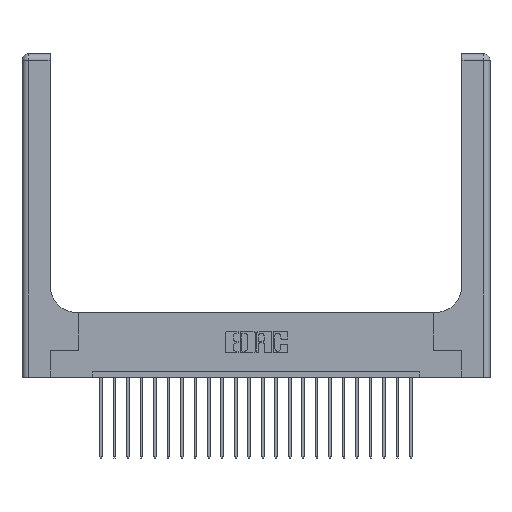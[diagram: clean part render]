
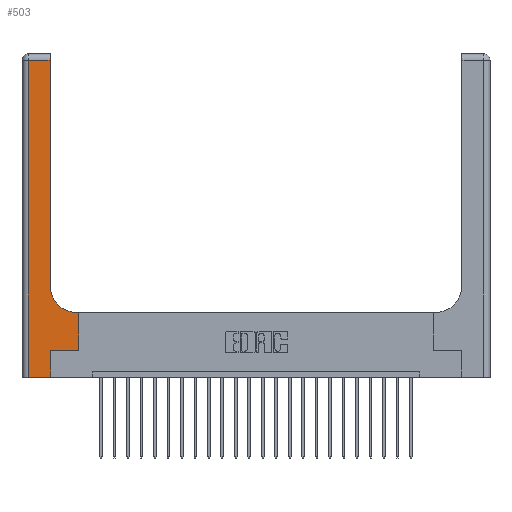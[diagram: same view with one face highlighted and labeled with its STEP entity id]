
A CAD part, top view. The second image highlights one B-rep face of the part: STEP entity #503.
In plain terms, the highlighted planar face has unit normal (0, 0, 1).
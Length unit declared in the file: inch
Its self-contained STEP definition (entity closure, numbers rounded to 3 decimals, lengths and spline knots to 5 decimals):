
#93 = LINE ( 'NONE', #9134, #2619 ) ;
#501 = FACE_OUTER_BOUND ( 'NONE', #10092, .T. ) ;
#503 = ADVANCED_FACE ( 'NONE', ( #501 ), #2582, .F. ) ;
#717 = VERTEX_POINT ( 'NONE', #13476 ) ;
#799 = ORIENTED_EDGE ( 'NONE', *, *, #3414, .T. ) ;
#1253 = CARTESIAN_POINT ( 'NONE',  ( 0.26, 2.94, 0.37 ) ) ;
#1261 = DIRECTION ( 'NONE',  ( 0., 1., 0. ) ) ;
#1490 = LINE ( 'NONE', #8557, #13143 ) ;
#2034 = VERTEX_POINT ( 'NONE', #3528 ) ;
#2071 = ORIENTED_EDGE ( 'NONE', *, *, #3049, .T. ) ;
#2171 = VECTOR ( 'NONE', #18870, 39.37008 ) ;
#2581 = VECTOR ( 'NONE', #14465, 39.37008 ) ;
#2582 = PLANE ( 'NONE',  #10431 ) ;
#2619 = VECTOR ( 'NONE', #10775, 39.37008 ) ;
#2918 = AXIS2_PLACEMENT_3D ( 'NONE', #22586, #13736, #18854 ) ;
#3049 = EDGE_CURVE ( 'NONE', #10993, #2034, #16896, .T. ) ;
#3401 = ORIENTED_EDGE ( 'NONE', *, *, #21704, .T. ) ;
#3414 = EDGE_CURVE ( 'NONE', #13813, #12497, #21888, .T. ) ;
#3528 = CARTESIAN_POINT ( 'NONE',  ( 0.06, 2.94, 0.37 ) ) ;
#3960 = EDGE_CURVE ( 'NONE', #717, #10993, #1490, .T. ) ;
#4150 = DIRECTION ( 'NONE',  ( 0., 1., 0. ) ) ;
#4334 = EDGE_CURVE ( 'NONE', #14161, #6647, #13865, .T. ) ;
#4589 = DIRECTION ( 'NONE',  ( 1., 0., 0. ) ) ;
#5173 = CARTESIAN_POINT ( 'NONE',  ( 0.265, 0., 0.37 ) ) ;
#5310 = ORIENTED_EDGE ( 'NONE', *, *, #20468, .T. ) ;
#5407 = CARTESIAN_POINT ( 'NONE',  ( 0.265, 0., 0.37 ) ) ;
#5960 = DIRECTION ( 'NONE',  ( -1., 0., 0. ) ) ;
#6062 = CARTESIAN_POINT ( 'NONE',  ( 0., 3., 0.37 ) ) ;
#6343 = ORIENTED_EDGE ( 'NONE', *, *, #11150, .T. ) ;
#6647 = VERTEX_POINT ( 'NONE', #16607 ) ;
#7266 = LINE ( 'NONE', #5407, #2581 ) ;
#7403 = CARTESIAN_POINT ( 'NONE',  ( 0.528, 0.25, 0.37 ) ) ;
#7699 = DIRECTION ( 'NONE',  ( -1., 0., 0. ) ) ;
#8183 = ORIENTED_EDGE ( 'NONE', *, *, #12344, .T. ) ;
#8557 = CARTESIAN_POINT ( 'NONE',  ( 0.26, 3., 0.37 ) ) ;
#8673 = VECTOR ( 'NONE', #4589, 39.37008 ) ;
#9134 = CARTESIAN_POINT ( 'NONE',  ( 0.06, 3., 0.37 ) ) ;
#9631 = DIRECTION ( 'NONE',  ( 1., 0., 0. ) ) ;
#9850 = LINE ( 'NONE', #10080, #19138 ) ;
#9871 = ORIENTED_EDGE ( 'NONE', *, *, #15803, .T. ) ;
#9935 = CARTESIAN_POINT ( 'NONE',  ( 0.265, 0.25, 0.37 ) ) ;
#10080 = CARTESIAN_POINT ( 'NONE',  ( 0., 0., 0.37 ) ) ;
#10092 = EDGE_LOOP ( 'NONE', ( #20943, #2071, #9871, #5310, #8183, #15857, #3401, #799, #6343 ) ) ;
#10431 = AXIS2_PLACEMENT_3D ( 'NONE', #6062, #22214, #7699 ) ;
#10775 = DIRECTION ( 'NONE',  ( 0., -1., 0. ) ) ;
#10993 = VERTEX_POINT ( 'NONE', #1253 ) ;
#11016 = VERTEX_POINT ( 'NONE', #5173 ) ;
#11150 = EDGE_CURVE ( 'NONE', #12497, #717, #12925, .T. ) ;
#12344 = EDGE_CURVE ( 'NONE', #11016, #14161, #7266, .T. ) ;
#12497 = VERTEX_POINT ( 'NONE', #16675 ) ;
#12925 = CIRCLE ( 'NONE', #2918, 0.25 ) ;
#13143 = VECTOR ( 'NONE', #1261, 39.37008 ) ;
#13476 = CARTESIAN_POINT ( 'NONE',  ( 0.26, 0.85, 0.37 ) ) ;
#13736 = DIRECTION ( 'NONE',  ( 0., 0., -1. ) ) ;
#13813 = VERTEX_POINT ( 'NONE', #18634 ) ;
#13865 = LINE ( 'NONE', #9935, #8673 ) ;
#14161 = VERTEX_POINT ( 'NONE', #20483 ) ;
#14440 = CARTESIAN_POINT ( 'NONE',  ( 0.26, 0.6, 0.37 ) ) ;
#14465 = DIRECTION ( 'NONE',  ( 0., 1., 0. ) ) ;
#15803 = EDGE_CURVE ( 'NONE', #2034, #19870, #93, .T. ) ;
#15857 = ORIENTED_EDGE ( 'NONE', *, *, #4334, .T. ) ;
#16607 = CARTESIAN_POINT ( 'NONE',  ( 0.528, 0.25, 0.37 ) ) ;
#16675 = CARTESIAN_POINT ( 'NONE',  ( 0.51, 0.6, 0.37 ) ) ;
#16896 = LINE ( 'NONE', #20620, #2171 ) ;
#18634 = CARTESIAN_POINT ( 'NONE',  ( 0.528, 0.6, 0.37 ) ) ;
#18718 = VECTOR ( 'NONE', #5960, 39.37008 ) ;
#18854 = DIRECTION ( 'NONE',  ( 1., 0., 0. ) ) ;
#18870 = DIRECTION ( 'NONE',  ( -1., 0., 0. ) ) ;
#19138 = VECTOR ( 'NONE', #9631, 39.37008 ) ;
#19870 = VERTEX_POINT ( 'NONE', #20010 ) ;
#20010 = CARTESIAN_POINT ( 'NONE',  ( 0.06, 0., 0.37 ) ) ;
#20468 = EDGE_CURVE ( 'NONE', #19870, #11016, #9850, .T. ) ;
#20483 = CARTESIAN_POINT ( 'NONE',  ( 0.265, 0.25, 0.37 ) ) ;
#20620 = CARTESIAN_POINT ( 'NONE',  ( 0., 2.94, 0.37 ) ) ;
#20943 = ORIENTED_EDGE ( 'NONE', *, *, #3960, .T. ) ;
#21690 = LINE ( 'NONE', #7403, #21777 ) ;
#21704 = EDGE_CURVE ( 'NONE', #6647, #13813, #21690, .T. ) ;
#21777 = VECTOR ( 'NONE', #4150, 39.37008 ) ;
#21888 = LINE ( 'NONE', #14440, #18718 ) ;
#22214 = DIRECTION ( 'NONE',  ( 0., 0., -1. ) ) ;
#22586 = CARTESIAN_POINT ( 'NONE',  ( 0.51, 0.85, 0.37 ) ) ;
